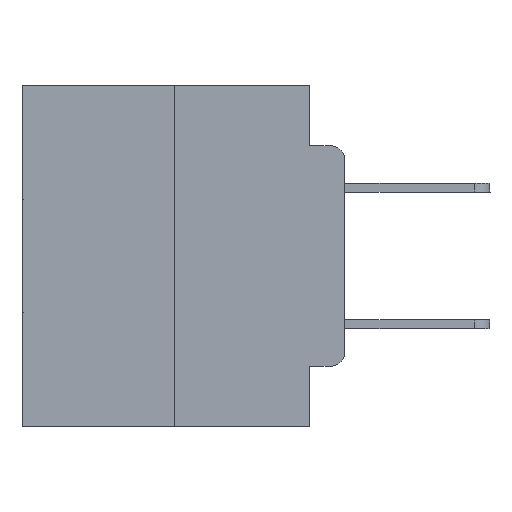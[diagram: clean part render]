
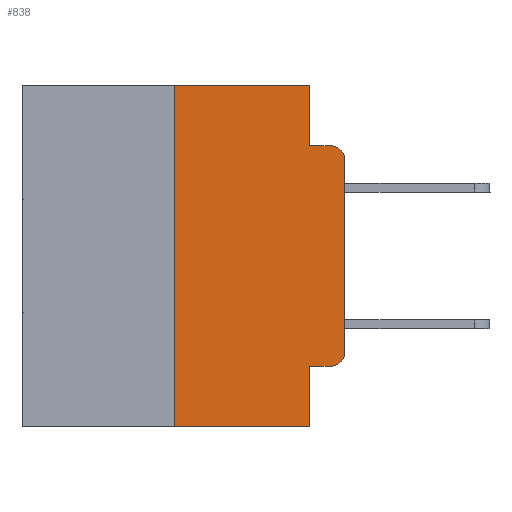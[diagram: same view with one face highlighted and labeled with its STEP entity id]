
A CAD part, left-side view. The second image highlights one B-rep face of the part: STEP entity #838.
In plain terms, the highlighted planar face has unit normal (-1, 0, 0).
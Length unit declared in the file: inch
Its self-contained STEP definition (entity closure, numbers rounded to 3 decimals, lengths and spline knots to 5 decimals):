
#45 = VECTOR ( 'NONE', #517, 39.37008 ) ;
#311 = VERTEX_POINT ( 'NONE', #19912 ) ;
#517 = DIRECTION ( 'NONE',  ( 0., 0., -1. ) ) ;
#838 = ADVANCED_FACE ( 'NONE', ( #6433 ), #5871, .F. ) ;
#856 = VERTEX_POINT ( 'NONE', #1277 ) ;
#1140 = DIRECTION ( 'NONE',  ( 0., 0., 1. ) ) ;
#1273 = DIRECTION ( 'NONE',  ( 0., -1., 0. ) ) ;
#1277 = CARTESIAN_POINT ( 'NONE',  ( 0., 0.25, -0.5 ) ) ;
#1366 = DIRECTION ( 'NONE',  ( 0., 0., 1. ) ) ;
#1466 = VECTOR ( 'NONE', #1366, 39.37008 ) ;
#1598 = LINE ( 'NONE', #22804, #12257 ) ;
#1733 = DIRECTION ( 'NONE',  ( -1., 0., 0. ) ) ;
#1937 = VECTOR ( 'NONE', #1273, 39.37008 ) ;
#2235 = EDGE_CURVE ( 'NONE', #311, #9621, #22721, .T. ) ;
#2528 = EDGE_CURVE ( 'NONE', #856, #11841, #12458, .T. ) ;
#2538 = VERTEX_POINT ( 'NONE', #28212 ) ;
#2871 = ORIENTED_EDGE ( 'NONE', *, *, #13169, .F. ) ;
#4316 = CARTESIAN_POINT ( 'NONE',  ( 0., 0., -0.3915 ) ) ;
#5066 = DIRECTION ( 'NONE',  ( 0., 0., -1. ) ) ;
#5871 = PLANE ( 'NONE',  #12329 ) ;
#6252 = CARTESIAN_POINT ( 'NONE',  ( 0., 0.02, -0.1085 ) ) ;
#6269 = ORIENTED_EDGE ( 'NONE', *, *, #27538, .T. ) ;
#6433 = FACE_OUTER_BOUND ( 'NONE', #23189, .T. ) ;
#6703 = ORIENTED_EDGE ( 'NONE', *, *, #27825, .F. ) ;
#6748 = EDGE_CURVE ( 'NONE', #11841, #11420, #28246, .T. ) ;
#7162 = CARTESIAN_POINT ( 'NONE',  ( 0., 0.051, -0.4115 ) ) ;
#7258 = CARTESIAN_POINT ( 'NONE',  ( 0., 0., -0.1085 ) ) ;
#7351 = VERTEX_POINT ( 'NONE', #4316 ) ;
#7801 = DIRECTION ( 'NONE',  ( -1., 0., 0. ) ) ;
#8096 = ORIENTED_EDGE ( 'NONE', *, *, #15250, .T. ) ;
#8237 = EDGE_CURVE ( 'NONE', #9621, #7351, #28092, .T. ) ;
#8492 = VECTOR ( 'NONE', #9135, 39.37008 ) ;
#8817 = DIRECTION ( 'NONE',  ( 0., 0., -1. ) ) ;
#9135 = DIRECTION ( 'NONE',  ( 0., -1., 0. ) ) ;
#9396 = LINE ( 'NONE', #12034, #26783 ) ;
#9451 = CARTESIAN_POINT ( 'NONE',  ( 0., 0.02, -0.0885 ) ) ;
#9621 = VERTEX_POINT ( 'NONE', #13916 ) ;
#11420 = VERTEX_POINT ( 'NONE', #21807 ) ;
#11723 = ORIENTED_EDGE ( 'NONE', *, *, #2235, .T. ) ;
#11841 = VERTEX_POINT ( 'NONE', #18166 ) ;
#12034 = CARTESIAN_POINT ( 'NONE',  ( 0., 0.051, 0. ) ) ;
#12106 = LINE ( 'NONE', #20727, #45 ) ;
#12257 = VECTOR ( 'NONE', #25052, 39.37008 ) ;
#12329 = AXIS2_PLACEMENT_3D ( 'NONE', #26299, #23735, #28601 ) ;
#12450 = CARTESIAN_POINT ( 'NONE',  ( 0., 0., 0. ) ) ;
#12454 = ORIENTED_EDGE ( 'NONE', *, *, #6748, .F. ) ;
#12458 = LINE ( 'NONE', #19405, #1466 ) ;
#13169 = EDGE_CURVE ( 'NONE', #28005, #14984, #1598, .T. ) ;
#13916 = CARTESIAN_POINT ( 'NONE',  ( 0., 0.02, -0.4115 ) ) ;
#14552 = AXIS2_PLACEMENT_3D ( 'NONE', #21409, #7801, #23665 ) ;
#14984 = VERTEX_POINT ( 'NONE', #9451 ) ;
#15127 = ORIENTED_EDGE ( 'NONE', *, *, #17542, .F. ) ;
#15250 = EDGE_CURVE ( 'NONE', #856, #2538, #16132, .T. ) ;
#16132 = LINE ( 'NONE', #17222, #1937 ) ;
#16493 = VECTOR ( 'NONE', #1140, 39.37008 ) ;
#17222 = CARTESIAN_POINT ( 'NONE',  ( 0., 0.473, -0.5 ) ) ;
#17542 = EDGE_CURVE ( 'NONE', #11420, #28005, #12106, .T. ) ;
#18166 = CARTESIAN_POINT ( 'NONE',  ( 0., 0.25, 0. ) ) ;
#19223 = VERTEX_POINT ( 'NONE', #7258 ) ;
#19405 = CARTESIAN_POINT ( 'NONE',  ( 0., 0.25, 0. ) ) ;
#19857 = ORIENTED_EDGE ( 'NONE', *, *, #8237, .T. ) ;
#19912 = CARTESIAN_POINT ( 'NONE',  ( 0., 0.051, -0.4115 ) ) ;
#20238 = CARTESIAN_POINT ( 'NONE',  ( 0., 0.051, -0.0885 ) ) ;
#20727 = CARTESIAN_POINT ( 'NONE',  ( 0., 0.051, 0. ) ) ;
#20925 = CARTESIAN_POINT ( 'NONE',  ( 0., 0.473, 0. ) ) ;
#21409 = CARTESIAN_POINT ( 'NONE',  ( 0., 0.02, -0.3915 ) ) ;
#21807 = CARTESIAN_POINT ( 'NONE',  ( 0., 0.051, 0. ) ) ;
#22115 = LINE ( 'NONE', #12450, #16493 ) ;
#22577 = VECTOR ( 'NONE', #23268, 39.37008 ) ;
#22721 = LINE ( 'NONE', #7162, #8492 ) ;
#22804 = CARTESIAN_POINT ( 'NONE',  ( 0., 0.051, -0.0885 ) ) ;
#23189 = EDGE_LOOP ( 'NONE', ( #24616, #6269, #2871, #15127, #12454, #24370, #8096, #6703, #11723, #19857 ) ) ;
#23268 = DIRECTION ( 'NONE',  ( 0., -1., 0. ) ) ;
#23304 = EDGE_CURVE ( 'NONE', #7351, #19223, #22115, .T. ) ;
#23665 = DIRECTION ( 'NONE',  ( 0., 0., -1. ) ) ;
#23735 = DIRECTION ( 'NONE',  ( 1., 0., 0. ) ) ;
#24300 = CIRCLE ( 'NONE', #27806, 0.02 ) ;
#24370 = ORIENTED_EDGE ( 'NONE', *, *, #2528, .F. ) ;
#24616 = ORIENTED_EDGE ( 'NONE', *, *, #23304, .T. ) ;
#25052 = DIRECTION ( 'NONE',  ( 0., -1., 0. ) ) ;
#26299 = CARTESIAN_POINT ( 'NONE',  ( 0., 0.473, 0. ) ) ;
#26783 = VECTOR ( 'NONE', #5066, 39.37008 ) ;
#27538 = EDGE_CURVE ( 'NONE', #19223, #14984, #24300, .T. ) ;
#27806 = AXIS2_PLACEMENT_3D ( 'NONE', #6252, #1733, #8817 ) ;
#27825 = EDGE_CURVE ( 'NONE', #311, #2538, #9396, .T. ) ;
#28005 = VERTEX_POINT ( 'NONE', #20238 ) ;
#28092 = CIRCLE ( 'NONE', #14552, 0.02 ) ;
#28212 = CARTESIAN_POINT ( 'NONE',  ( 0., 0.051, -0.5 ) ) ;
#28246 = LINE ( 'NONE', #20925, #22577 ) ;
#28601 = DIRECTION ( 'NONE',  ( 0., 0., -1. ) ) ;
